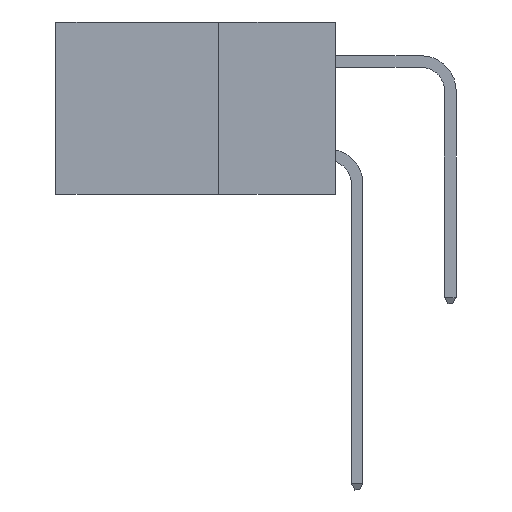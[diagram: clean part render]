
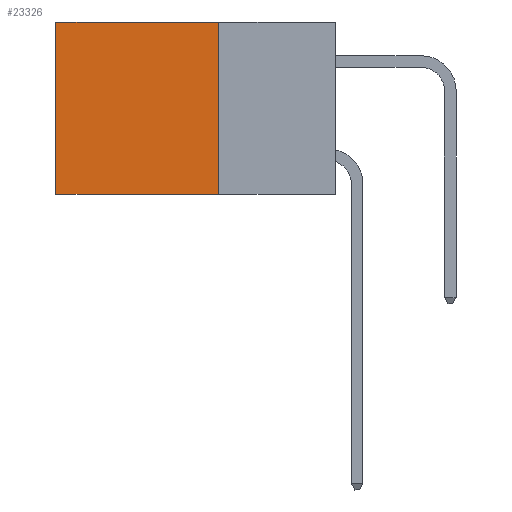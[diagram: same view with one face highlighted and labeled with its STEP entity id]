
A CAD part, left-side view. The second image highlights one B-rep face of the part: STEP entity #23326.
In plain terms, the highlighted planar face has unit normal (-1, 0, 0).
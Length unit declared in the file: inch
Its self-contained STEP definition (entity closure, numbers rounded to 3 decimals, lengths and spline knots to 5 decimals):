
#1191 = CARTESIAN_POINT ( 'NONE',  ( 0.2875, 0.25, 0. ) ) ;
#2274 = AXIS2_PLACEMENT_3D ( 'NONE', #23217, #8431, #25595 ) ;
#2924 = EDGE_CURVE ( 'NONE', #15773, #16085, #6895, .T. ) ;
#3447 = ORIENTED_EDGE ( 'NONE', *, *, #11618, .T. ) ;
#5868 = PLANE ( 'NONE',  #2274 ) ;
#6895 = LINE ( 'NONE', #23905, #25742 ) ;
#6991 = ORIENTED_EDGE ( 'NONE', *, *, #15266, .F. ) ;
#7694 = CARTESIAN_POINT ( 'NONE',  ( 0.2875, 0.25, 0. ) ) ;
#8431 = DIRECTION ( 'NONE',  ( 1., 0., 0. ) ) ;
#10571 = EDGE_LOOP ( 'NONE', ( #24211, #31505, #6991, #3447 ) ) ;
#10805 = VECTOR ( 'NONE', #27280, 39.37008 ) ;
#11174 = VECTOR ( 'NONE', #21199, 39.37008 ) ;
#11618 = EDGE_CURVE ( 'NONE', #31049, #15773, #30556, .T. ) ;
#12765 = VERTEX_POINT ( 'NONE', #25613 ) ;
#15266 = EDGE_CURVE ( 'NONE', #31049, #12765, #18149, .T. ) ;
#15773 = VERTEX_POINT ( 'NONE', #19829 ) ;
#15993 = CARTESIAN_POINT ( 'NONE',  ( 0.2875, 0.25, 0. ) ) ;
#16085 = VERTEX_POINT ( 'NONE', #28472 ) ;
#16672 = DIRECTION ( 'NONE',  ( 0., 0., -1. ) ) ;
#18149 = LINE ( 'NONE', #7694, #10805 ) ;
#19070 = LINE ( 'NONE', #20137, #30341 ) ;
#19829 = CARTESIAN_POINT ( 'NONE',  ( 0.2875, 0.6, 0. ) ) ;
#20137 = CARTESIAN_POINT ( 'NONE',  ( 0.2875, 0.25, -0.37 ) ) ;
#21199 = DIRECTION ( 'NONE',  ( 0., 1., 0. ) ) ;
#23217 = CARTESIAN_POINT ( 'NONE',  ( 0.2875, 0.25, 0. ) ) ;
#23326 = ADVANCED_FACE ( 'NONE', ( #26331 ), #5868, .F. ) ;
#23905 = CARTESIAN_POINT ( 'NONE',  ( 0.2875, 0.6, 0. ) ) ;
#24211 = ORIENTED_EDGE ( 'NONE', *, *, #2924, .T. ) ;
#25256 = EDGE_CURVE ( 'NONE', #12765, #16085, #19070, .T. ) ;
#25595 = DIRECTION ( 'NONE',  ( 0., 0., -1. ) ) ;
#25613 = CARTESIAN_POINT ( 'NONE',  ( 0.2875, 0.25, -0.37 ) ) ;
#25742 = VECTOR ( 'NONE', #16672, 39.37008 ) ;
#26331 = FACE_OUTER_BOUND ( 'NONE', #10571, .T. ) ;
#27280 = DIRECTION ( 'NONE',  ( 0., 0., -1. ) ) ;
#27352 = DIRECTION ( 'NONE',  ( 0., 1., 0. ) ) ;
#28472 = CARTESIAN_POINT ( 'NONE',  ( 0.2875, 0.6, -0.37 ) ) ;
#30341 = VECTOR ( 'NONE', #27352, 39.37008 ) ;
#30556 = LINE ( 'NONE', #1191, #11174 ) ;
#31049 = VERTEX_POINT ( 'NONE', #15993 ) ;
#31505 = ORIENTED_EDGE ( 'NONE', *, *, #25256, .F. ) ;
